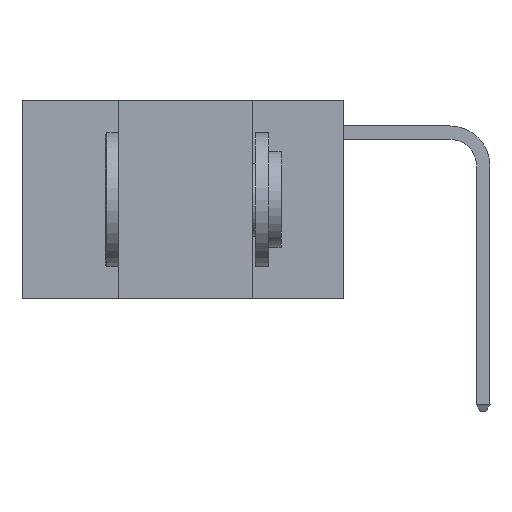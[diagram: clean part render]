
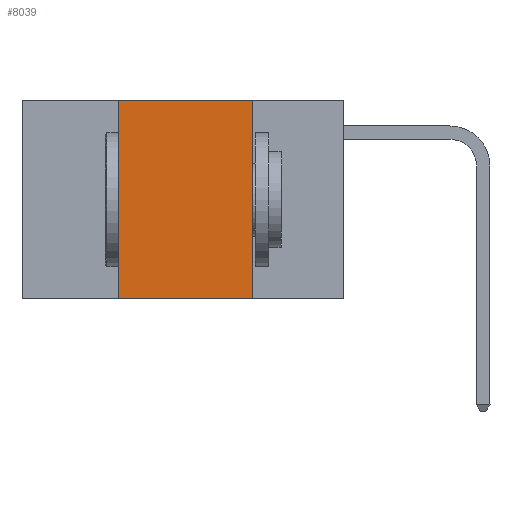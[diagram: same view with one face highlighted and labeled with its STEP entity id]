
A CAD part, left-side view. The second image highlights one B-rep face of the part: STEP entity #8039.
In plain terms, the highlighted planar face has unit normal (-1, 0, 0).
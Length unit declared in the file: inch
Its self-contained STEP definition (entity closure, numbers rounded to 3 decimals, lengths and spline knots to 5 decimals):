
#1045 = DIRECTION ( 'NONE',  ( 0., 0., -1. ) ) ;
#1179 = VERTEX_POINT ( 'NONE', #6651 ) ;
#2500 = DIRECTION ( 'NONE',  ( 0., 0., 1. ) ) ;
#3401 = ORIENTED_EDGE ( 'NONE', *, *, #3890, .F. ) ;
#3486 = VECTOR ( 'NONE', #2500, 39.37008 ) ;
#3488 = ORIENTED_EDGE ( 'NONE', *, *, #5808, .F. ) ;
#3890 = EDGE_CURVE ( 'NONE', #1179, #11602, #4278, .T. ) ;
#4278 = LINE ( 'NONE', #11750, #3486 ) ;
#5083 = CARTESIAN_POINT ( 'NONE',  ( 0., 0.17, -0.37 ) ) ;
#5808 = EDGE_CURVE ( 'NONE', #11602, #15562, #10653, .T. ) ;
#6572 = FACE_OUTER_BOUND ( 'NONE', #16622, .T. ) ;
#6601 = CARTESIAN_POINT ( 'NONE',  ( 0., 0.42, 0. ) ) ;
#6651 = CARTESIAN_POINT ( 'NONE',  ( 0., 0.42, -0.37 ) ) ;
#6984 = CARTESIAN_POINT ( 'NONE',  ( 0., 0.6, 0. ) ) ;
#8039 = ADVANCED_FACE ( 'NONE', ( #6572 ), #12004, .F. ) ;
#10291 = EDGE_CURVE ( 'NONE', #15562, #21812, #11733, .T. ) ;
#10306 = LINE ( 'NONE', #11842, #13183 ) ;
#10386 = VECTOR ( 'NONE', #14201, 39.37008 ) ;
#10653 = LINE ( 'NONE', #6984, #10386 ) ;
#11270 = ORIENTED_EDGE ( 'NONE', *, *, #22794, .T. ) ;
#11602 = VERTEX_POINT ( 'NONE', #6601 ) ;
#11733 = LINE ( 'NONE', #20909, #11985 ) ;
#11750 = CARTESIAN_POINT ( 'NONE',  ( 0., 0.42, 0. ) ) ;
#11842 = CARTESIAN_POINT ( 'NONE',  ( 0., 0.6, -0.37 ) ) ;
#11985 = VECTOR ( 'NONE', #1045, 39.37008 ) ;
#12004 = PLANE ( 'NONE',  #21483 ) ;
#12030 = CARTESIAN_POINT ( 'NONE',  ( 0., 0.17, 0. ) ) ;
#13183 = VECTOR ( 'NONE', #19006, 39.37008 ) ;
#14201 = DIRECTION ( 'NONE',  ( 0., -1., 0. ) ) ;
#15562 = VERTEX_POINT ( 'NONE', #12030 ) ;
#15805 = DIRECTION ( 'NONE',  ( 0., 0., -1. ) ) ;
#15955 = ORIENTED_EDGE ( 'NONE', *, *, #10291, .F. ) ;
#16622 = EDGE_LOOP ( 'NONE', ( #15955, #3488, #3401, #11270 ) ) ;
#17487 = DIRECTION ( 'NONE',  ( 1., 0., 0. ) ) ;
#19006 = DIRECTION ( 'NONE',  ( 0., -1., 0. ) ) ;
#19279 = CARTESIAN_POINT ( 'NONE',  ( 0., 0.6, 0. ) ) ;
#20909 = CARTESIAN_POINT ( 'NONE',  ( 0., 0.17, 0. ) ) ;
#21483 = AXIS2_PLACEMENT_3D ( 'NONE', #19279, #17487, #15805 ) ;
#21812 = VERTEX_POINT ( 'NONE', #5083 ) ;
#22794 = EDGE_CURVE ( 'NONE', #1179, #21812, #10306, .T. ) ;
